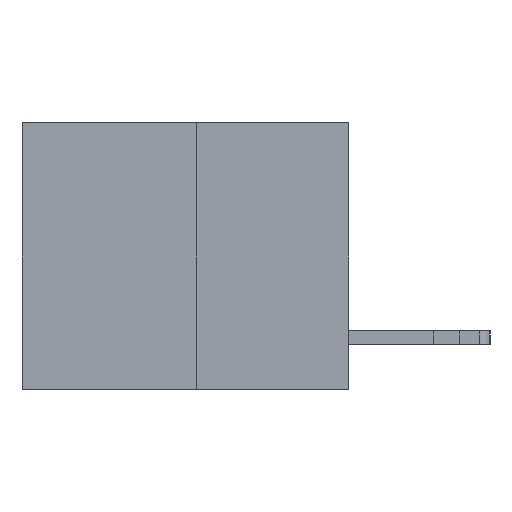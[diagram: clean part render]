
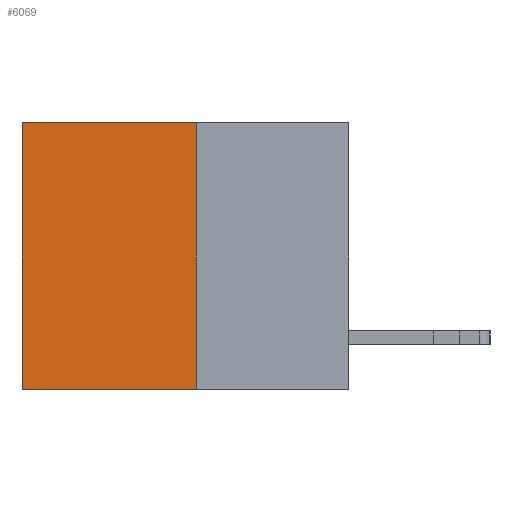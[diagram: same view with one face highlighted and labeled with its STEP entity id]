
A CAD part, left-side view. The second image highlights one B-rep face of the part: STEP entity #6069.
In plain terms, the highlighted planar face has unit normal (-1, 0, 0).
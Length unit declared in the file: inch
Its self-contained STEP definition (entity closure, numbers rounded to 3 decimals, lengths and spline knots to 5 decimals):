
#870 = VECTOR ( 'NONE', #17369, 39.37008 ) ;
#1251 = DIRECTION ( 'NONE',  ( 0., 0., -1. ) ) ;
#1369 = ORIENTED_EDGE ( 'NONE', *, *, #15995, .F. ) ;
#2408 = LINE ( 'NONE', #8042, #16511 ) ;
#4181 = VERTEX_POINT ( 'NONE', #13836 ) ;
#5224 = VERTEX_POINT ( 'NONE', #6991 ) ;
#6069 = ADVANCED_FACE ( 'NONE', ( #7608 ), #7300, .F. ) ;
#6991 = CARTESIAN_POINT ( 'NONE',  ( 0.3165, 0.28, 0. ) ) ;
#7300 = PLANE ( 'NONE',  #7519 ) ;
#7327 = CARTESIAN_POINT ( 'NONE',  ( 0.3165, 0.6, -0.49 ) ) ;
#7519 = AXIS2_PLACEMENT_3D ( 'NONE', #8780, #7743, #8723 ) ;
#7608 = FACE_OUTER_BOUND ( 'NONE', #12979, .T. ) ;
#7743 = DIRECTION ( 'NONE',  ( 1., 0., 0. ) ) ;
#8042 = CARTESIAN_POINT ( 'NONE',  ( 0.3165, 0.28, 0. ) ) ;
#8146 = VERTEX_POINT ( 'NONE', #18778 ) ;
#8357 = LINE ( 'NONE', #18513, #9272 ) ;
#8549 = DIRECTION ( 'NONE',  ( 0., 1., 0. ) ) ;
#8683 = CARTESIAN_POINT ( 'NONE',  ( 0.3165, 0.28, -0.49 ) ) ;
#8723 = DIRECTION ( 'NONE',  ( 0., 0., -1. ) ) ;
#8780 = CARTESIAN_POINT ( 'NONE',  ( 0.3165, 0.28, -0.49 ) ) ;
#9272 = VECTOR ( 'NONE', #1251, 39.37008 ) ;
#9505 = DIRECTION ( 'NONE',  ( 0., 1., 0. ) ) ;
#10130 = EDGE_CURVE ( 'NONE', #4181, #12444, #17293, .T. ) ;
#10825 = EDGE_CURVE ( 'NONE', #5224, #4181, #2408, .T. ) ;
#12084 = ORIENTED_EDGE ( 'NONE', *, *, #10825, .T. ) ;
#12208 = CARTESIAN_POINT ( 'NONE',  ( 0.3165, 0.6, -0.49 ) ) ;
#12444 = VERTEX_POINT ( 'NONE', #12208 ) ;
#12979 = EDGE_LOOP ( 'NONE', ( #15379, #15544, #1369, #12084 ) ) ;
#13428 = EDGE_CURVE ( 'NONE', #8146, #12444, #18128, .T. ) ;
#13836 = CARTESIAN_POINT ( 'NONE',  ( 0.3165, 0.6, 0. ) ) ;
#15379 = ORIENTED_EDGE ( 'NONE', *, *, #10130, .T. ) ;
#15544 = ORIENTED_EDGE ( 'NONE', *, *, #13428, .F. ) ;
#15995 = EDGE_CURVE ( 'NONE', #5224, #8146, #8357, .T. ) ;
#16511 = VECTOR ( 'NONE', #9505, 39.37008 ) ;
#16767 = VECTOR ( 'NONE', #8549, 39.37008 ) ;
#17293 = LINE ( 'NONE', #7327, #870 ) ;
#17369 = DIRECTION ( 'NONE',  ( 0., 0., -1. ) ) ;
#18128 = LINE ( 'NONE', #8683, #16767 ) ;
#18513 = CARTESIAN_POINT ( 'NONE',  ( 0.3165, 0.28, -0.49 ) ) ;
#18778 = CARTESIAN_POINT ( 'NONE',  ( 0.3165, 0.28, -0.49 ) ) ;
